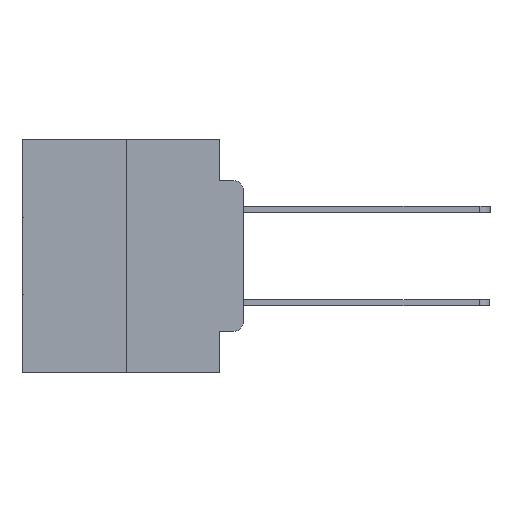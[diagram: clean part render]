
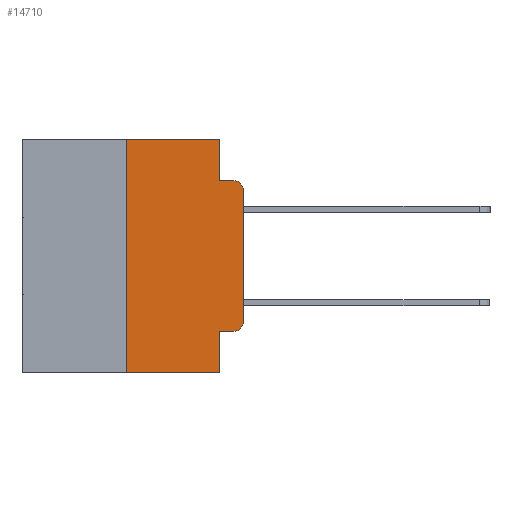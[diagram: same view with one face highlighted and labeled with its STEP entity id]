
A CAD part, left-side view. The second image highlights one B-rep face of the part: STEP entity #14710.
In plain terms, the highlighted planar face has unit normal (-1, 0, 0).
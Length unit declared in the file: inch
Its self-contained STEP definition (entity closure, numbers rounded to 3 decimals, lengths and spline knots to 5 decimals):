
#192 = VERTEX_POINT ( 'NONE', #21501 ) ;
#536 = ORIENTED_EDGE ( 'NONE', *, *, #3011, .F. ) ;
#719 = DIRECTION ( 'NONE',  ( 0., 0., 1. ) ) ;
#793 = VERTEX_POINT ( 'NONE', #21540 ) ;
#924 = CARTESIAN_POINT ( 'NONE',  ( 0., 0.051, 0. ) ) ;
#947 = CARTESIAN_POINT ( 'NONE',  ( 0., 0.02, -0.3915 ) ) ;
#1239 = VECTOR ( 'NONE', #28283, 39.37008 ) ;
#1393 = EDGE_CURVE ( 'NONE', #26943, #17135, #3138, .T. ) ;
#1880 = VECTOR ( 'NONE', #7283, 39.37008 ) ;
#2382 = DIRECTION ( 'NONE',  ( 0., 0., -1. ) ) ;
#2622 = CARTESIAN_POINT ( 'NONE',  ( 0., 0.051, 0. ) ) ;
#2790 = CARTESIAN_POINT ( 'NONE',  ( 0., 0.25, -0.5 ) ) ;
#3011 = EDGE_CURVE ( 'NONE', #17135, #192, #19856, .T. ) ;
#3138 = LINE ( 'NONE', #24128, #14479 ) ;
#3263 = CARTESIAN_POINT ( 'NONE',  ( 0., 0.02, -0.0885 ) ) ;
#3717 = VECTOR ( 'NONE', #18933, 39.37008 ) ;
#3837 = AXIS2_PLACEMENT_3D ( 'NONE', #25906, #12799, #28106 ) ;
#4474 = EDGE_CURVE ( 'NONE', #9181, #5335, #27660, .T. ) ;
#4658 = VERTEX_POINT ( 'NONE', #16706 ) ;
#4825 = VERTEX_POINT ( 'NONE', #14972 ) ;
#5076 = VECTOR ( 'NONE', #28556, 39.37008 ) ;
#5335 = VERTEX_POINT ( 'NONE', #3263 ) ;
#6015 = EDGE_CURVE ( 'NONE', #28107, #5335, #13461, .T. ) ;
#6182 = VERTEX_POINT ( 'NONE', #6185 ) ;
#6185 = CARTESIAN_POINT ( 'NONE',  ( 0., 0.02, -0.4115 ) ) ;
#6383 = EDGE_LOOP ( 'NONE', ( #16870, #12254, #18293, #7581, #536, #15335, #20232, #9865, #28461, #22144 ) ) ;
#6750 = CARTESIAN_POINT ( 'NONE',  ( 0., 0.473, 0. ) ) ;
#7283 = DIRECTION ( 'NONE',  ( 0., -1., 0. ) ) ;
#7581 = ORIENTED_EDGE ( 'NONE', *, *, #24403, .F. ) ;
#8652 = CARTESIAN_POINT ( 'NONE',  ( 0., 0., 0. ) ) ;
#9181 = VERTEX_POINT ( 'NONE', #25965 ) ;
#9865 = ORIENTED_EDGE ( 'NONE', *, *, #23079, .F. ) ;
#10783 = EDGE_CURVE ( 'NONE', #26943, #793, #12511, .T. ) ;
#11086 = LINE ( 'NONE', #8652, #5076 ) ;
#11256 = DIRECTION ( 'NONE',  ( 0., -1., 0. ) ) ;
#11560 = CARTESIAN_POINT ( 'NONE',  ( 0., 0.02, -0.1085 ) ) ;
#12025 = CARTESIAN_POINT ( 'NONE',  ( 0., 0.25, 0. ) ) ;
#12254 = ORIENTED_EDGE ( 'NONE', *, *, #4474, .T. ) ;
#12511 = LINE ( 'NONE', #22760, #1880 ) ;
#12799 = DIRECTION ( 'NONE',  ( 1., 0., 0. ) ) ;
#12973 = CARTESIAN_POINT ( 'NONE',  ( 0., 0.051, -0.4115 ) ) ;
#13333 = VECTOR ( 'NONE', #11256, 39.37008 ) ;
#13461 = LINE ( 'NONE', #25686, #15562 ) ;
#13550 = EDGE_CURVE ( 'NONE', #4825, #9181, #11086, .T. ) ;
#13819 = DIRECTION ( 'NONE',  ( 0., 0., -1. ) ) ;
#14014 = CARTESIAN_POINT ( 'NONE',  ( 0., 0.051, -0.0885 ) ) ;
#14237 = AXIS2_PLACEMENT_3D ( 'NONE', #947, #15914, #2382 ) ;
#14479 = VECTOR ( 'NONE', #719, 39.37008 ) ;
#14623 = DIRECTION ( 'NONE',  ( 0., -1., 0. ) ) ;
#14710 = ADVANCED_FACE ( 'NONE', ( #26120 ), #21552, .F. ) ;
#14972 = CARTESIAN_POINT ( 'NONE',  ( 0., 0., -0.3915 ) ) ;
#15335 = ORIENTED_EDGE ( 'NONE', *, *, #1393, .F. ) ;
#15562 = VECTOR ( 'NONE', #14623, 39.37008 ) ;
#15782 = EDGE_CURVE ( 'NONE', #6182, #4825, #22007, .T. ) ;
#15914 = DIRECTION ( 'NONE',  ( -1., 0., 0. ) ) ;
#16103 = VECTOR ( 'NONE', #18331, 39.37008 ) ;
#16706 = CARTESIAN_POINT ( 'NONE',  ( 0., 0.051, -0.4115 ) ) ;
#16870 = ORIENTED_EDGE ( 'NONE', *, *, #13550, .T. ) ;
#17135 = VERTEX_POINT ( 'NONE', #12025 ) ;
#18293 = ORIENTED_EDGE ( 'NONE', *, *, #6015, .F. ) ;
#18331 = DIRECTION ( 'NONE',  ( 0., 0., -1. ) ) ;
#18933 = DIRECTION ( 'NONE',  ( 0., 0., -1. ) ) ;
#19856 = LINE ( 'NONE', #6750, #13333 ) ;
#20232 = ORIENTED_EDGE ( 'NONE', *, *, #10783, .T. ) ;
#21458 = EDGE_CURVE ( 'NONE', #4658, #6182, #22938, .T. ) ;
#21501 = CARTESIAN_POINT ( 'NONE',  ( 0., 0.051, 0. ) ) ;
#21540 = CARTESIAN_POINT ( 'NONE',  ( 0., 0.051, -0.5 ) ) ;
#21552 = PLANE ( 'NONE',  #3837 ) ;
#22007 = CIRCLE ( 'NONE', #14237, 0.02 ) ;
#22144 = ORIENTED_EDGE ( 'NONE', *, *, #15782, .T. ) ;
#22760 = CARTESIAN_POINT ( 'NONE',  ( 0., 0.473, -0.5 ) ) ;
#22938 = LINE ( 'NONE', #12973, #1239 ) ;
#23079 = EDGE_CURVE ( 'NONE', #4658, #793, #26618, .T. ) ;
#24128 = CARTESIAN_POINT ( 'NONE',  ( 0., 0.25, 0. ) ) ;
#24403 = EDGE_CURVE ( 'NONE', #192, #28107, #27019, .T. ) ;
#25686 = CARTESIAN_POINT ( 'NONE',  ( 0., 0.051, -0.0885 ) ) ;
#25906 = CARTESIAN_POINT ( 'NONE',  ( 0., 0.473, 0. ) ) ;
#25965 = CARTESIAN_POINT ( 'NONE',  ( 0., 0., -0.1085 ) ) ;
#26120 = FACE_OUTER_BOUND ( 'NONE', #6383, .T. ) ;
#26618 = LINE ( 'NONE', #924, #3717 ) ;
#26915 = DIRECTION ( 'NONE',  ( -1., 0., 0. ) ) ;
#26943 = VERTEX_POINT ( 'NONE', #2790 ) ;
#27019 = LINE ( 'NONE', #2622, #16103 ) ;
#27660 = CIRCLE ( 'NONE', #28133, 0.02 ) ;
#28106 = DIRECTION ( 'NONE',  ( 0., 0., -1. ) ) ;
#28107 = VERTEX_POINT ( 'NONE', #14014 ) ;
#28133 = AXIS2_PLACEMENT_3D ( 'NONE', #11560, #26915, #13819 ) ;
#28283 = DIRECTION ( 'NONE',  ( 0., -1., 0. ) ) ;
#28461 = ORIENTED_EDGE ( 'NONE', *, *, #21458, .T. ) ;
#28556 = DIRECTION ( 'NONE',  ( 0., 0., 1. ) ) ;
